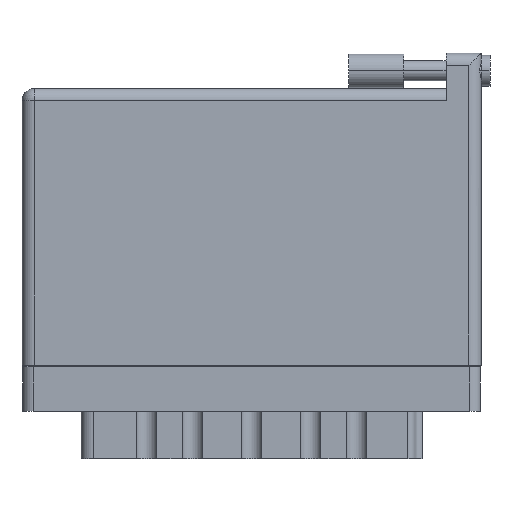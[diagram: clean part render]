
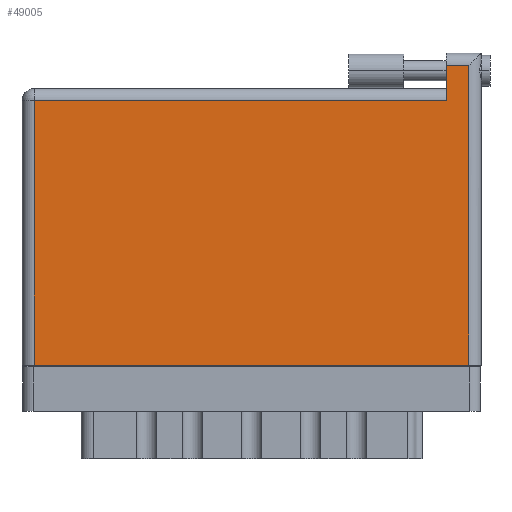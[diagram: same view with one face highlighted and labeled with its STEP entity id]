
A CAD part, front view. The second image highlights one B-rep face of the part: STEP entity #49005.
In plain terms, the highlighted face is planar.
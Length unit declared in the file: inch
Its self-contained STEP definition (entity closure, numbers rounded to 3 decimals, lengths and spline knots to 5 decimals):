
#541 = VECTOR ( 'NONE', #37302, 39.37008 ) ;
#1062 = EDGE_CURVE ( 'NONE', #3349, #34339, #20837, .T. ) ;
#2005 = ORIENTED_EDGE ( 'NONE', *, *, #32281, .T. ) ;
#3019 = DIRECTION ( 'NONE',  ( 1., 0., 0. ) ) ;
#3349 = VERTEX_POINT ( 'NONE', #9353 ) ;
#3688 = VECTOR ( 'NONE', #42988, 39.37008 ) ;
#5041 = DIRECTION ( 'NONE',  ( -1., 0., 0. ) ) ;
#5508 = CARTESIAN_POINT ( 'NONE',  ( 2.403, 1.496, 0. ) ) ;
#5998 = DIRECTION ( 'NONE',  ( 0., -1., 0. ) ) ;
#6262 = LINE ( 'NONE', #21948, #33050 ) ;
#8400 = LINE ( 'NONE', #25684, #541 ) ;
#8846 = AXIS2_PLACEMENT_3D ( 'NONE', #12416, #41302, #20765 ) ;
#8981 = EDGE_CURVE ( 'NONE', #29639, #3349, #17364, .T. ) ;
#9353 = CARTESIAN_POINT ( 'NONE',  ( 0.07, 1.496, 0. ) ) ;
#10911 = CARTESIAN_POINT ( 'NONE',  ( 0.07, 0., 0. ) ) ;
#11947 = CARTESIAN_POINT ( 'NONE',  ( 0.07, 0., 0. ) ) ;
#12416 = CARTESIAN_POINT ( 'NONE',  ( 0., 1.566, 0. ) ) ;
#13567 = EDGE_CURVE ( 'NONE', #17656, #31230, #21526, .T. ) ;
#15269 = ORIENTED_EDGE ( 'NONE', *, *, #13567, .T. ) ;
#16944 = VERTEX_POINT ( 'NONE', #35981 ) ;
#17364 = LINE ( 'NONE', #47036, #3688 ) ;
#17656 = VERTEX_POINT ( 'NONE', #34729 ) ;
#20765 = DIRECTION ( 'NONE',  ( -1., 0., 0. ) ) ;
#20837 = LINE ( 'NONE', #11947, #29207 ) ;
#21526 = LINE ( 'NONE', #41257, #42999 ) ;
#21948 = CARTESIAN_POINT ( 'NONE',  ( 2.403, 1.766, 0. ) ) ;
#23833 = CARTESIAN_POINT ( 'NONE',  ( 0., 0., 0. ) ) ;
#24076 = VECTOR ( 'NONE', #3019, 39.37008 ) ;
#25684 = CARTESIAN_POINT ( 'NONE',  ( 2.53, 1.766, 0. ) ) ;
#27268 = EDGE_CURVE ( 'NONE', #34339, #16944, #28162, .T. ) ;
#27519 = ORIENTED_EDGE ( 'NONE', *, *, #8981, .T. ) ;
#28162 = LINE ( 'NONE', #23833, #24076 ) ;
#28425 = DIRECTION ( 'NONE',  ( 0., -1., 0. ) ) ;
#29207 = VECTOR ( 'NONE', #28425, 39.37008 ) ;
#29639 = VERTEX_POINT ( 'NONE', #5508 ) ;
#31230 = VERTEX_POINT ( 'NONE', #35301 ) ;
#31957 = ORIENTED_EDGE ( 'NONE', *, *, #1062, .T. ) ;
#32281 = EDGE_CURVE ( 'NONE', #31230, #29639, #6262, .T. ) ;
#33050 = VECTOR ( 'NONE', #5998, 39.37008 ) ;
#34339 = VERTEX_POINT ( 'NONE', #10911 ) ;
#34729 = CARTESIAN_POINT ( 'NONE',  ( 2.53, 1.696, 0. ) ) ;
#35301 = CARTESIAN_POINT ( 'NONE',  ( 2.403, 1.696, 0. ) ) ;
#35981 = CARTESIAN_POINT ( 'NONE',  ( 2.53, 0., 0. ) ) ;
#37295 = EDGE_CURVE ( 'NONE', #16944, #17656, #8400, .T. ) ;
#37302 = DIRECTION ( 'NONE',  ( 0., 1., 0. ) ) ;
#41257 = CARTESIAN_POINT ( 'NONE',  ( 0., 1.696, 0. ) ) ;
#41302 = DIRECTION ( 'NONE',  ( 0., 0., -1. ) ) ;
#42220 = ORIENTED_EDGE ( 'NONE', *, *, #27268, .T. ) ;
#42988 = DIRECTION ( 'NONE',  ( -1., 0., 0. ) ) ;
#42999 = VECTOR ( 'NONE', #5041, 39.37008 ) ;
#46325 = EDGE_LOOP ( 'NONE', ( #42220, #47126, #15269, #2005, #27519, #31957 ) ) ;
#47036 = CARTESIAN_POINT ( 'NONE',  ( 0., 1.496, 0. ) ) ;
#47126 = ORIENTED_EDGE ( 'NONE', *, *, #37295, .T. ) ;
#49005 = ADVANCED_FACE ( 'NONE', ( #53178 ), #49121, .F. ) ;
#49121 = PLANE ( 'NONE',  #8846 ) ;
#53178 = FACE_OUTER_BOUND ( 'NONE', #46325, .T. ) ;
